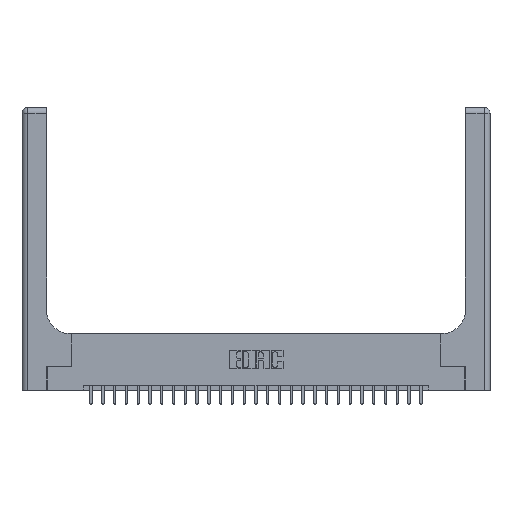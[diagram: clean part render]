
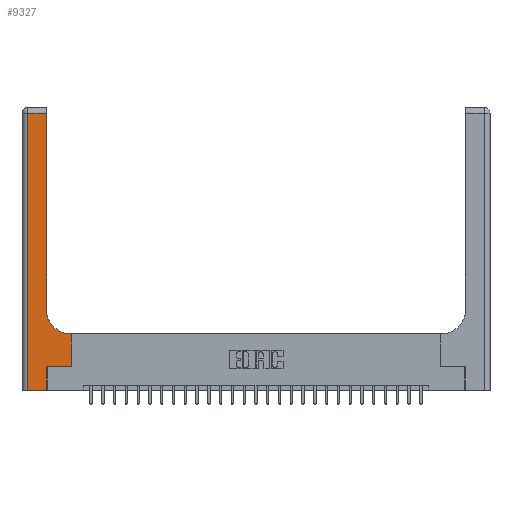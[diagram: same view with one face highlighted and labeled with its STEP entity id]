
A CAD part, top view. The second image highlights one B-rep face of the part: STEP entity #9327.
In plain terms, the highlighted planar face has unit normal (0, 0, 1).
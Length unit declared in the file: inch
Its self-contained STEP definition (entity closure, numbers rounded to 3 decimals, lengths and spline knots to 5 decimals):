
#377 = ORIENTED_EDGE ( 'NONE', *, *, #16917, .T. ) ;
#386 = DIRECTION ( 'NONE',  ( 0., 1., 0. ) ) ;
#993 = VERTEX_POINT ( 'NONE', #13084 ) ;
#1538 = CARTESIAN_POINT ( 'NONE',  ( 0., 0., 0.37 ) ) ;
#1703 = CARTESIAN_POINT ( 'NONE',  ( 0.265, 0., 0.37 ) ) ;
#1706 = CIRCLE ( 'NONE', #6422, 0.25 ) ;
#1722 = VECTOR ( 'NONE', #15301, 39.37008 ) ;
#1971 = EDGE_CURVE ( 'NONE', #6216, #15688, #8563, .T. ) ;
#1973 = EDGE_CURVE ( 'NONE', #24203, #24746, #18575, .T. ) ;
#2195 = CARTESIAN_POINT ( 'NONE',  ( 0., 2.94, 0.37 ) ) ;
#2577 = VECTOR ( 'NONE', #14878, 39.37008 ) ;
#2829 = DIRECTION ( 'NONE',  ( 0., 0., -1. ) ) ;
#2915 = VECTOR ( 'NONE', #25324, 39.37008 ) ;
#3448 = FACE_OUTER_BOUND ( 'NONE', #17337, .T. ) ;
#3493 = VECTOR ( 'NONE', #12992, 39.37008 ) ;
#3543 = LINE ( 'NONE', #7523, #2915 ) ;
#3640 = VECTOR ( 'NONE', #386, 39.37008 ) ;
#3776 = EDGE_CURVE ( 'NONE', #24746, #15176, #3543, .T. ) ;
#3847 = ORIENTED_EDGE ( 'NONE', *, *, #24213, .T. ) ;
#3941 = LINE ( 'NONE', #2195, #13947 ) ;
#4661 = ORIENTED_EDGE ( 'NONE', *, *, #16689, .T. ) ;
#4791 = DIRECTION ( 'NONE',  ( -1., 0., 0. ) ) ;
#5620 = EDGE_CURVE ( 'NONE', #15176, #993, #23612, .T. ) ;
#5668 = ORIENTED_EDGE ( 'NONE', *, *, #1971, .T. ) ;
#6044 = VECTOR ( 'NONE', #10789, 39.37008 ) ;
#6216 = VERTEX_POINT ( 'NONE', #11205 ) ;
#6422 = AXIS2_PLACEMENT_3D ( 'NONE', #24670, #2829, #8805 ) ;
#6476 = LINE ( 'NONE', #15703, #3640 ) ;
#6505 = VECTOR ( 'NONE', #21486, 39.37008 ) ;
#7523 = CARTESIAN_POINT ( 'NONE',  ( 0.528, 0.25, 0.37 ) ) ;
#7923 = CARTESIAN_POINT ( 'NONE',  ( 0.26, 0.85, 0.37 ) ) ;
#8232 = EDGE_CURVE ( 'NONE', #21959, #11788, #20690, .T. ) ;
#8485 = ORIENTED_EDGE ( 'NONE', *, *, #13148, .T. ) ;
#8563 = LINE ( 'NONE', #16719, #6044 ) ;
#8805 = DIRECTION ( 'NONE',  ( 1., 0., 0. ) ) ;
#9327 = ADVANCED_FACE ( 'NONE', ( #3448 ), #12900, .F. ) ;
#10789 = DIRECTION ( 'NONE',  ( 0., -1., 0. ) ) ;
#11205 = CARTESIAN_POINT ( 'NONE',  ( 0.06, 2.94, 0.37 ) ) ;
#11788 = VERTEX_POINT ( 'NONE', #21717 ) ;
#12900 = PLANE ( 'NONE',  #14756 ) ;
#12992 = DIRECTION ( 'NONE',  ( 0., 1., 0. ) ) ;
#13084 = CARTESIAN_POINT ( 'NONE',  ( 0.51, 0.6, 0.37 ) ) ;
#13148 = EDGE_CURVE ( 'NONE', #993, #21959, #1706, .T. ) ;
#13947 = VECTOR ( 'NONE', #21898, 39.37008 ) ;
#14756 = AXIS2_PLACEMENT_3D ( 'NONE', #18640, #22609, #4791 ) ;
#14878 = DIRECTION ( 'NONE',  ( 1., 0., 0. ) ) ;
#15176 = VERTEX_POINT ( 'NONE', #25581 ) ;
#15301 = DIRECTION ( 'NONE',  ( -1., 0., 0. ) ) ;
#15688 = VERTEX_POINT ( 'NONE', #21141 ) ;
#15693 = ORIENTED_EDGE ( 'NONE', *, *, #8232, .T. ) ;
#15703 = CARTESIAN_POINT ( 'NONE',  ( 0.265, 0., 0.37 ) ) ;
#16689 = EDGE_CURVE ( 'NONE', #15688, #22608, #19916, .T. ) ;
#16719 = CARTESIAN_POINT ( 'NONE',  ( 0.06, 3., 0.37 ) ) ;
#16917 = EDGE_CURVE ( 'NONE', #22608, #24203, #6476, .T. ) ;
#16946 = ORIENTED_EDGE ( 'NONE', *, *, #5620, .T. ) ;
#17337 = EDGE_LOOP ( 'NONE', ( #15693, #3847, #5668, #4661, #377, #18306, #22882, #16946, #8485 ) ) ;
#18306 = ORIENTED_EDGE ( 'NONE', *, *, #1973, .T. ) ;
#18575 = LINE ( 'NONE', #22816, #2577 ) ;
#18640 = CARTESIAN_POINT ( 'NONE',  ( 0., 3., 0.37 ) ) ;
#19916 = LINE ( 'NONE', #1538, #6505 ) ;
#20690 = LINE ( 'NONE', #23129, #3493 ) ;
#21137 = CARTESIAN_POINT ( 'NONE',  ( 0.265, 0.25, 0.37 ) ) ;
#21141 = CARTESIAN_POINT ( 'NONE',  ( 0.06, 0., 0.37 ) ) ;
#21486 = DIRECTION ( 'NONE',  ( 1., 0., 0. ) ) ;
#21717 = CARTESIAN_POINT ( 'NONE',  ( 0.26, 2.94, 0.37 ) ) ;
#21898 = DIRECTION ( 'NONE',  ( -1., 0., 0. ) ) ;
#21959 = VERTEX_POINT ( 'NONE', #7923 ) ;
#22608 = VERTEX_POINT ( 'NONE', #1703 ) ;
#22609 = DIRECTION ( 'NONE',  ( 0., 0., -1. ) ) ;
#22816 = CARTESIAN_POINT ( 'NONE',  ( 0.265, 0.25, 0.37 ) ) ;
#22882 = ORIENTED_EDGE ( 'NONE', *, *, #3776, .T. ) ;
#23129 = CARTESIAN_POINT ( 'NONE',  ( 0.26, 3., 0.37 ) ) ;
#23335 = CARTESIAN_POINT ( 'NONE',  ( 0.26, 0.6, 0.37 ) ) ;
#23612 = LINE ( 'NONE', #23335, #1722 ) ;
#24203 = VERTEX_POINT ( 'NONE', #21137 ) ;
#24213 = EDGE_CURVE ( 'NONE', #11788, #6216, #3941, .T. ) ;
#24376 = CARTESIAN_POINT ( 'NONE',  ( 0.528, 0.25, 0.37 ) ) ;
#24670 = CARTESIAN_POINT ( 'NONE',  ( 0.51, 0.85, 0.37 ) ) ;
#24746 = VERTEX_POINT ( 'NONE', #24376 ) ;
#25324 = DIRECTION ( 'NONE',  ( 0., 1., 0. ) ) ;
#25581 = CARTESIAN_POINT ( 'NONE',  ( 0.528, 0.6, 0.37 ) ) ;
